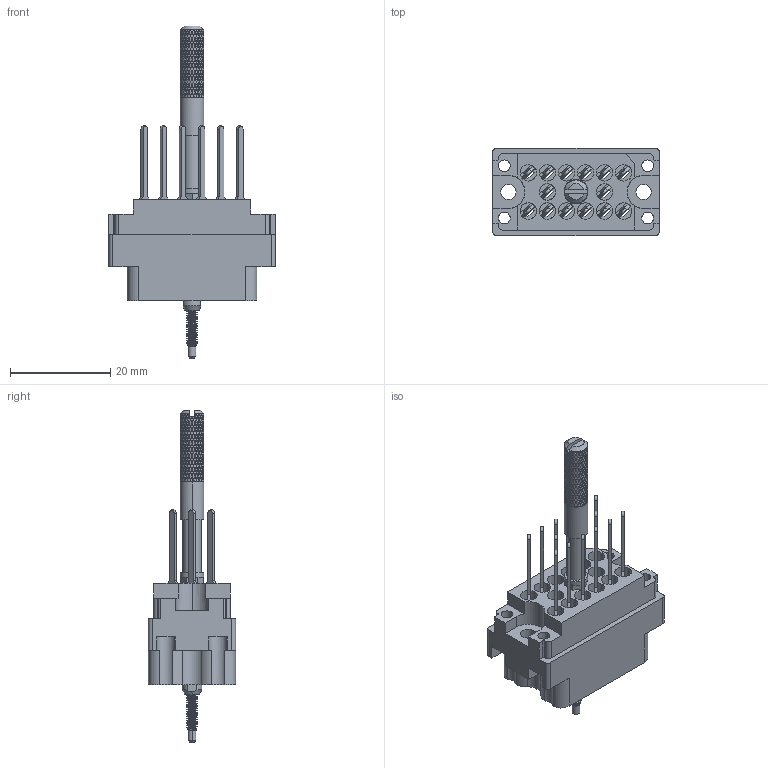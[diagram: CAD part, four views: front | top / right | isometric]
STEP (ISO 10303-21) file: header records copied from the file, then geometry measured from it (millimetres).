
FILE_DESCRIPTION (( 'STEP AP203' ), '1' );
FILE_NAME ('519-014-540-305.STEP', '2020-03-02T21:00:43', ( '' ), ( '' ), 'SwSTEP 2.0', 'SolidWorks 2016', '' );
FILE_SCHEMA (( 'CONFIG_CONTROL_DESIGN' ));
Length unit declared in the file: inch
Products named in the file (9): 516-250-020-111; 516-251-025-100; 519-014-540-305; 519 Plug Insulator_014; 516-250-021-102_519; 516-292-001_540 Contact; 516-252-022-102; Actuating Screw Assy 020; 516-253-025-100
Assembly tree (21 placements, depth 3):
  519-014-540-305
    519 Plug Insulator_014
    516-292-001_540 Contact  x14
    Actuating Screw Assy 020
      516-251-025-100
      516-250-021-102_519
      516-250-020-111
      516-253-025-100
      516-252-022-102
Bounding box: 33.32 x 17.42 x 66.29 mm (x, y, z)
Volume: 6319.3 mm3; surface area: 10286.4 mm2
Topology: 20 solids, 20 shells, 4180 faces, 9914 edges, 5788 vertices
Faces by surface type: bspline 2106, cylinder 1061, plane 993, cone 20
Entity records: 178153 total; most frequent: CARTESIAN_POINT 128567, ORIENTED_EDGE 14420, EDGE_CURVE 7210, DIRECTION 4930, VERTEX_POINT 3994, EDGE_LOOP 3310, FACE_OUTER_BOUND 3244, ADVANCED_FACE 3244
